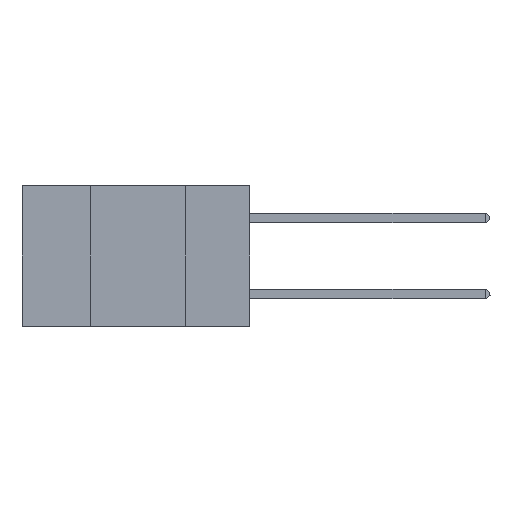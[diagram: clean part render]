
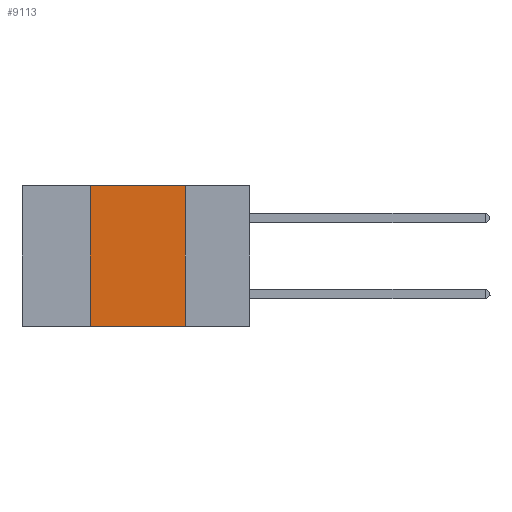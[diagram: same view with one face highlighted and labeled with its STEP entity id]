
A CAD part, left-side view. The second image highlights one B-rep face of the part: STEP entity #9113.
In plain terms, the highlighted planar face has unit normal (-1, 0, 0).
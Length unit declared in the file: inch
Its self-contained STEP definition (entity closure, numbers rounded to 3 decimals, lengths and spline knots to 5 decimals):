
#179 = ORIENTED_EDGE ( 'NONE', *, *, #31855, .F. ) ;
#819 = EDGE_LOOP ( 'NONE', ( #179, #21876, #13076, #11247 ) ) ;
#1836 = CARTESIAN_POINT ( 'NONE',  ( 0., 0.42, -0.37 ) ) ;
#5429 = EDGE_CURVE ( 'NONE', #26185, #22853, #42322, .T. ) ;
#5685 = EDGE_CURVE ( 'NONE', #33252, #12367, #24533, .T. ) ;
#7004 = VECTOR ( 'NONE', #42996, 39.37008 ) ;
#7272 = DIRECTION ( 'NONE',  ( 0., 0., -1. ) ) ;
#9113 = ADVANCED_FACE ( 'NONE', ( #44337 ), #25250, .F. ) ;
#9297 = CARTESIAN_POINT ( 'NONE',  ( 0., 0.17, -0.37 ) ) ;
#11247 = ORIENTED_EDGE ( 'NONE', *, *, #5685, .T. ) ;
#12367 = VERTEX_POINT ( 'NONE', #9297 ) ;
#13076 = ORIENTED_EDGE ( 'NONE', *, *, #27359, .F. ) ;
#14879 = VECTOR ( 'NONE', #43618, 39.37008 ) ;
#14928 = VECTOR ( 'NONE', #23474, 39.37008 ) ;
#16228 = CARTESIAN_POINT ( 'NONE',  ( 0., 0.6, -0.37 ) ) ;
#19857 = CARTESIAN_POINT ( 'NONE',  ( 0., 0.6, 0. ) ) ;
#21876 = ORIENTED_EDGE ( 'NONE', *, *, #5429, .F. ) ;
#22853 = VERTEX_POINT ( 'NONE', #30586 ) ;
#23474 = DIRECTION ( 'NONE',  ( 0., -1., 0. ) ) ;
#24533 = LINE ( 'NONE', #16228, #14928 ) ;
#25250 = PLANE ( 'NONE',  #40260 ) ;
#26185 = VERTEX_POINT ( 'NONE', #44773 ) ;
#26475 = VECTOR ( 'NONE', #44106, 39.37008 ) ;
#27359 = EDGE_CURVE ( 'NONE', #33252, #26185, #35469, .T. ) ;
#28640 = DIRECTION ( 'NONE',  ( 1., 0., 0. ) ) ;
#30586 = CARTESIAN_POINT ( 'NONE',  ( 0., 0.17, 0. ) ) ;
#31855 = EDGE_CURVE ( 'NONE', #22853, #12367, #34047, .T. ) ;
#33252 = VERTEX_POINT ( 'NONE', #1836 ) ;
#34047 = LINE ( 'NONE', #39610, #7004 ) ;
#35469 = LINE ( 'NONE', #40707, #26475 ) ;
#39610 = CARTESIAN_POINT ( 'NONE',  ( 0., 0.17, 0. ) ) ;
#40260 = AXIS2_PLACEMENT_3D ( 'NONE', #45294, #28640, #7272 ) ;
#40707 = CARTESIAN_POINT ( 'NONE',  ( 0., 0.42, 0. ) ) ;
#42322 = LINE ( 'NONE', #19857, #14879 ) ;
#42996 = DIRECTION ( 'NONE',  ( 0., 0., -1. ) ) ;
#43618 = DIRECTION ( 'NONE',  ( 0., -1., 0. ) ) ;
#44106 = DIRECTION ( 'NONE',  ( 0., 0., 1. ) ) ;
#44337 = FACE_OUTER_BOUND ( 'NONE', #819, .T. ) ;
#44773 = CARTESIAN_POINT ( 'NONE',  ( 0., 0.42, 0. ) ) ;
#45294 = CARTESIAN_POINT ( 'NONE',  ( 0., 0.6, 0. ) ) ;
